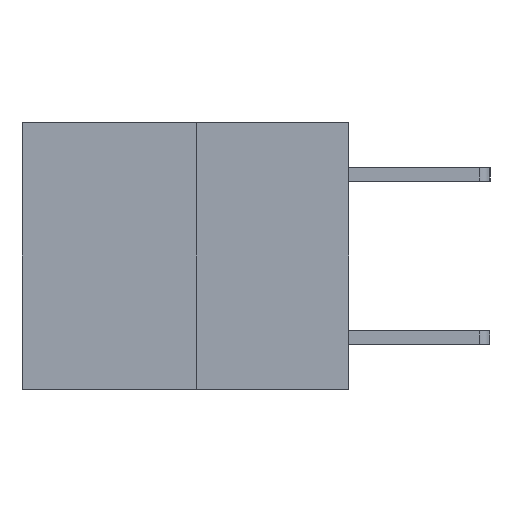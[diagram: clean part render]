
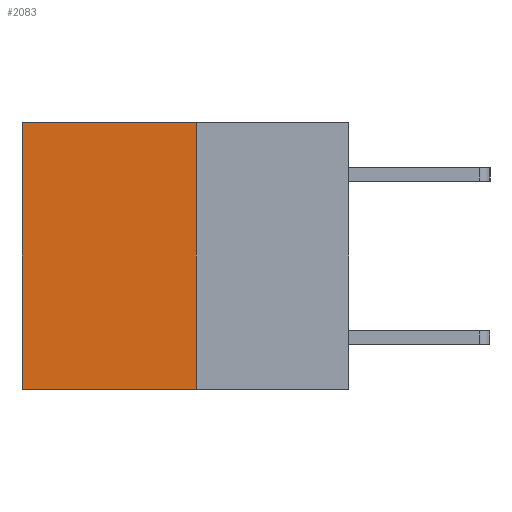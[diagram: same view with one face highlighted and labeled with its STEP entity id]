
A CAD part, left-side view. The second image highlights one B-rep face of the part: STEP entity #2083.
In plain terms, the highlighted planar face has unit normal (-1, 0, 0).
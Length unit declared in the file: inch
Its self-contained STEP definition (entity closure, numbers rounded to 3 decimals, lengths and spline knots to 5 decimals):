
#125 = AXIS2_PLACEMENT_3D ( 'NONE', #6676, #10583, #1162 ) ;
#141 = ORIENTED_EDGE ( 'NONE', *, *, #6346, .F. ) ;
#182 = VECTOR ( 'NONE', #5534, 39.37008 ) ;
#1016 = DIRECTION ( 'NONE',  ( 0., 1., 0. ) ) ;
#1162 = DIRECTION ( 'NONE',  ( 0., 0., -1. ) ) ;
#1241 = PLANE ( 'NONE',  #125 ) ;
#1616 = ORIENTED_EDGE ( 'NONE', *, *, #6713, .T. ) ;
#2083 = ADVANCED_FACE ( 'NONE', ( #11618 ), #1241, .F. ) ;
#3430 = CARTESIAN_POINT ( 'NONE',  ( 0.3165, 0.6, -0.49 ) ) ;
#5448 = CARTESIAN_POINT ( 'NONE',  ( 0.3165, 0.28, -0.49 ) ) ;
#5449 = DIRECTION ( 'NONE',  ( 0., 0., -1. ) ) ;
#5534 = DIRECTION ( 'NONE',  ( 0., 0., -1. ) ) ;
#5679 = EDGE_LOOP ( 'NONE', ( #11310, #141, #7155, #1616 ) ) ;
#5951 = CARTESIAN_POINT ( 'NONE',  ( 0.3165, 0.6, 0. ) ) ;
#6026 = VECTOR ( 'NONE', #1016, 39.37008 ) ;
#6234 = CARTESIAN_POINT ( 'NONE',  ( 0.3165, 0.28, -0.49 ) ) ;
#6346 = EDGE_CURVE ( 'NONE', #6612, #8823, #11306, .T. ) ;
#6612 = VERTEX_POINT ( 'NONE', #6234 ) ;
#6676 = CARTESIAN_POINT ( 'NONE',  ( 0.3165, 0.28, -0.49 ) ) ;
#6713 = EDGE_CURVE ( 'NONE', #7385, #10155, #9392, .T. ) ;
#7150 = LINE ( 'NONE', #11015, #8030 ) ;
#7155 = ORIENTED_EDGE ( 'NONE', *, *, #7538, .F. ) ;
#7385 = VERTEX_POINT ( 'NONE', #10941 ) ;
#7538 = EDGE_CURVE ( 'NONE', #7385, #6612, #9072, .T. ) ;
#8030 = VECTOR ( 'NONE', #5449, 39.37008 ) ;
#8035 = CARTESIAN_POINT ( 'NONE',  ( 0.3165, 0.28, 0. ) ) ;
#8526 = CARTESIAN_POINT ( 'NONE',  ( 0.3165, 0.28, -0.49 ) ) ;
#8823 = VERTEX_POINT ( 'NONE', #3430 ) ;
#9072 = LINE ( 'NONE', #5448, #182 ) ;
#9392 = LINE ( 'NONE', #8035, #11011 ) ;
#9960 = DIRECTION ( 'NONE',  ( 0., 1., 0. ) ) ;
#10155 = VERTEX_POINT ( 'NONE', #5951 ) ;
#10583 = DIRECTION ( 'NONE',  ( 1., 0., 0. ) ) ;
#10799 = EDGE_CURVE ( 'NONE', #10155, #8823, #7150, .T. ) ;
#10941 = CARTESIAN_POINT ( 'NONE',  ( 0.3165, 0.28, 0. ) ) ;
#11011 = VECTOR ( 'NONE', #9960, 39.37008 ) ;
#11015 = CARTESIAN_POINT ( 'NONE',  ( 0.3165, 0.6, -0.49 ) ) ;
#11306 = LINE ( 'NONE', #8526, #6026 ) ;
#11310 = ORIENTED_EDGE ( 'NONE', *, *, #10799, .T. ) ;
#11618 = FACE_OUTER_BOUND ( 'NONE', #5679, .T. ) ;
